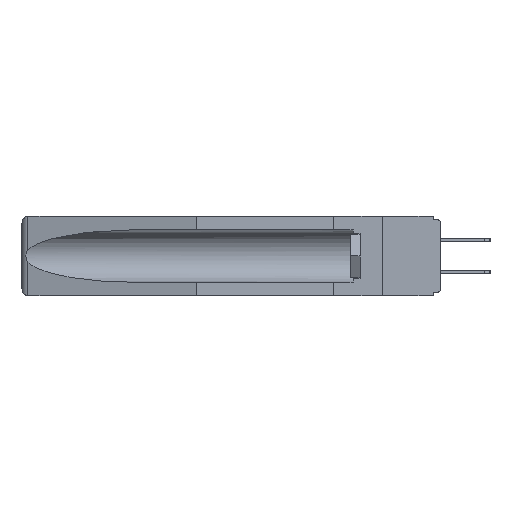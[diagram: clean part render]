
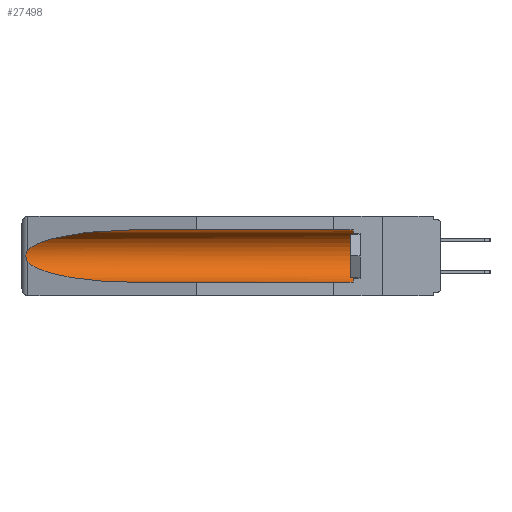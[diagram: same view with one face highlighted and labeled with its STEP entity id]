
A CAD part, left-side view. The second image highlights one B-rep face of the part: STEP entity #27498.
In plain terms, the highlighted cylindrical face has radius 2.857 mm (diameter 5.715 mm), a partial arc.
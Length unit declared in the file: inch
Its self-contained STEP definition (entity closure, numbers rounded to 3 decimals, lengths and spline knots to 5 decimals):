
#100 = CARTESIAN_POINT ( 'NONE',  ( 0.26597, 1.52961, -0.15275 ) ) ;
#598 = EDGE_LOOP ( 'NONE', ( #11893, #2840, #2121, #6914, #13666, #4031 ) ) ;
#809 = CARTESIAN_POINT ( 'NONE',  ( 0.155, 0.126, -0.284 ) ) ;
#1636 = CARTESIAN_POINT ( 'NONE',  ( 0.21114, 1.30732, -0.284 ) ) ;
#2121 = ORIENTED_EDGE ( 'NONE', *, *, #19914, .T. ) ;
#2307 = CARTESIAN_POINT ( 'NONE',  ( 0.2675, 1.53308, -0.16763 ) ) ;
#2505 = CARTESIAN_POINT ( 'NONE',  ( 0.26654, 1.53092, -0.15636 ) ) ;
#2599 = CARTESIAN_POINT ( 'NONE',  ( 0.155, 0.126, -0.059 ) ) ;
#2840 = ORIENTED_EDGE ( 'NONE', *, *, #12141, .T. ) ;
#3138 = DIRECTION ( 'NONE',  ( 0., 1., 0. ) ) ;
#4031 = ORIENTED_EDGE ( 'NONE', *, *, #18941, .T. ) ;
#4344 = LINE ( 'NONE', #24156, #16093 ) ;
#4900 = CARTESIAN_POINT ( 'NONE',  ( 0.2673, 1.5327, -0.16383 ) ) ;
#5473 = DIRECTION ( 'NONE',  ( 0., 1., 0. ) ) ;
#5515 = CARTESIAN_POINT ( 'NONE',  ( 0.26537, 1.52718, -0.19328 ) ) ;
#6465 = AXIS2_PLACEMENT_3D ( 'NONE', #22551, #29675, #8643 ) ;
#6508 = CARTESIAN_POINT ( 'NONE',  ( 0.26537, 1.52718, -0.19328 ) ) ;
#6877 = CARTESIAN_POINT ( 'NONE',  ( 0.155, 1.07973, -0.059 ) ) ;
#6914 = ORIENTED_EDGE ( 'NONE', *, *, #7171, .F. ) ;
#6974 = CARTESIAN_POINT ( 'NONE',  ( 0.26537, 1.52718, -0.14972 ) ) ;
#7072 = DIRECTION ( 'NONE',  ( 0., 0., 1. ) ) ;
#7131 = VERTEX_POINT ( 'NONE', #2599 ) ;
#7171 = EDGE_CURVE ( 'NONE', #25857, #30334, #10835, .T. ) ;
#8575 = CARTESIAN_POINT ( 'NONE',  ( 0.155, 1.07973, -0.284 ) ) ;
#8643 = DIRECTION ( 'NONE',  ( 0., 0., 1. ) ) ;
#8824 = VERTEX_POINT ( 'NONE', #19326 ) ;
#8954 =( BOUNDED_CURVE ( )  B_SPLINE_CURVE ( 3, ( #6508, #22867, #1636, #30015 ),
 .UNSPECIFIED., .F., .F. ) 
 B_SPLINE_CURVE_WITH_KNOTS ( ( 4, 4 ),
 ( 0.1948, 1.5708 ),
 .UNSPECIFIED. ) 
 CURVE ( )  GEOMETRIC_REPRESENTATION_ITEM ( )  RATIONAL_B_SPLINE_CURVE ( ( 1., 0.848, 0.848, 1. ) ) 
 REPRESENTATION_ITEM ( '' )  );
#10269 = B_SPLINE_CURVE_WITH_KNOTS ( 'NONE', 3,
 ( #14253, #100, #2505, #4900, #2307, #25731, #14151, #25827, #11683, #5515 ),
 .UNSPECIFIED., .F., .F.,
 ( 4, 2, 2, 2, 4 ),
 ( 0., 0.00029, 0.00058, 0.00087, 0.00117 ),
 .UNSPECIFIED. ) ;
#10835 = LINE ( 'NONE', #19506, #26271 ) ;
#11683 = CARTESIAN_POINT ( 'NONE',  ( 0.26597, 1.5296, -0.19026 ) ) ;
#11893 = ORIENTED_EDGE ( 'NONE', *, *, #29914, .T. ) ;
#12141 = EDGE_CURVE ( 'NONE', #12263, #8824, #10269, .T. ) ;
#12220 = FACE_OUTER_BOUND ( 'NONE', #598, .T. ) ;
#12263 = VERTEX_POINT ( 'NONE', #14927 ) ;
#13666 = ORIENTED_EDGE ( 'NONE', *, *, #28049, .T. ) ;
#14061 = CARTESIAN_POINT ( 'NONE',  ( 0.155, 1.07973, -0.059 ) ) ;
#14151 = CARTESIAN_POINT ( 'NONE',  ( 0.2673, 1.53269, -0.17917 ) ) ;
#14164 = CARTESIAN_POINT ( 'NONE',  ( 0.21114, 1.30732, -0.059 ) ) ;
#14253 = CARTESIAN_POINT ( 'NONE',  ( 0.26537, 1.52718, -0.14972 ) ) ;
#14927 = CARTESIAN_POINT ( 'NONE',  ( 0.26537, 1.52718, -0.14972 ) ) ;
#16093 = VECTOR ( 'NONE', #3138, 39.37008 ) ;
#17704 = VERTEX_POINT ( 'NONE', #6877 ) ;
#17764 =( BOUNDED_CURVE ( )  B_SPLINE_CURVE ( 3, ( #14061, #14164, #18656, #6974 ),
 .UNSPECIFIED., .F., .T. ) 
 B_SPLINE_CURVE_WITH_KNOTS ( ( 4, 4 ),
 ( 4.71239, 6.08839 ),
 .UNSPECIFIED. ) 
 CURVE ( )  GEOMETRIC_REPRESENTATION_ITEM ( )  RATIONAL_B_SPLINE_CURVE ( ( 1., 0.848, 0.848, 1. ) ) 
 REPRESENTATION_ITEM ( '' )  );
#18656 = CARTESIAN_POINT ( 'NONE',  ( 0.25451, 1.48313, -0.09465 ) ) ;
#18941 = EDGE_CURVE ( 'NONE', #7131, #17704, #4344, .T. ) ;
#19326 = CARTESIAN_POINT ( 'NONE',  ( 0.26537, 1.52718, -0.19328 ) ) ;
#19506 = CARTESIAN_POINT ( 'NONE',  ( 0.155, -0.30754, -0.284 ) ) ;
#19914 = EDGE_CURVE ( 'NONE', #8824, #30334, #8954, .T. ) ;
#21097 = CARTESIAN_POINT ( 'NONE',  ( 0.155, 0.126, -0.1715 ) ) ;
#22391 = AXIS2_PLACEMENT_3D ( 'NONE', #21097, #27815, #7072 ) ;
#22551 = CARTESIAN_POINT ( 'NONE',  ( 0.155, -0.30754, -0.1715 ) ) ;
#22867 = CARTESIAN_POINT ( 'NONE',  ( 0.25451, 1.48313, -0.24835 ) ) ;
#24156 = CARTESIAN_POINT ( 'NONE',  ( 0.155, -0.30754, -0.059 ) ) ;
#25731 = CARTESIAN_POINT ( 'NONE',  ( 0.2675, 1.53308, -0.17534 ) ) ;
#25827 = CARTESIAN_POINT ( 'NONE',  ( 0.26655, 1.53094, -0.18657 ) ) ;
#25857 = VERTEX_POINT ( 'NONE', #809 ) ;
#26271 = VECTOR ( 'NONE', #5473, 39.37008 ) ;
#27498 = ADVANCED_FACE ( 'NONE', ( #12220 ), #28015, .F. ) ;
#27815 = DIRECTION ( 'NONE',  ( 0., -1., 0. ) ) ;
#28015 = CYLINDRICAL_SURFACE ( 'NONE', #6465, 0.1125 ) ;
#28049 = EDGE_CURVE ( 'NONE', #25857, #7131, #29792, .T. ) ;
#29675 = DIRECTION ( 'NONE',  ( 0., 1., 0. ) ) ;
#29792 = CIRCLE ( 'NONE', #22391, 0.1125 ) ;
#29914 = EDGE_CURVE ( 'NONE', #17704, #12263, #17764, .T. ) ;
#30015 = CARTESIAN_POINT ( 'NONE',  ( 0.155, 1.07973, -0.284 ) ) ;
#30334 = VERTEX_POINT ( 'NONE', #8575 ) ;
